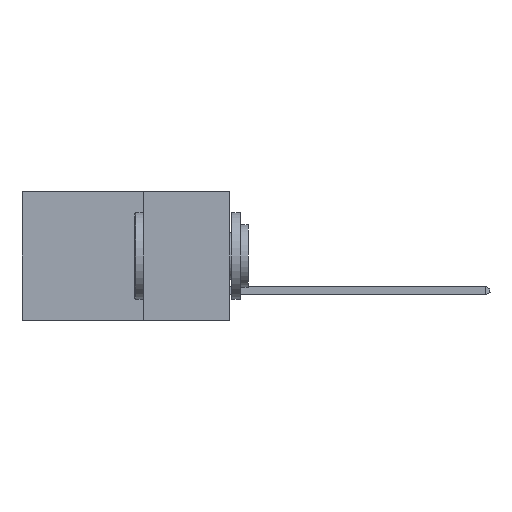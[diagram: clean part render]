
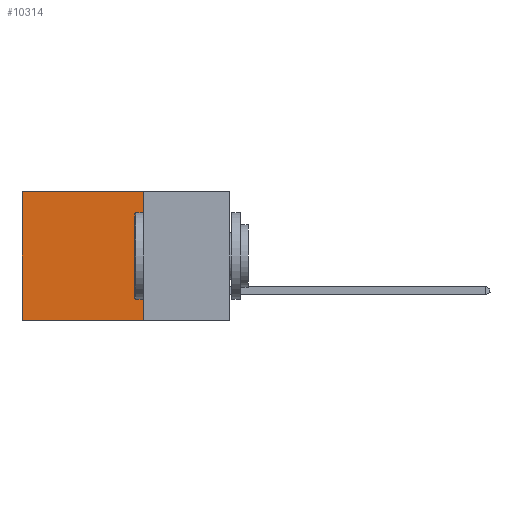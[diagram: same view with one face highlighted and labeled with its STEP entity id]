
A CAD part, left-side view. The second image highlights one B-rep face of the part: STEP entity #10314.
In plain terms, the highlighted planar face has unit normal (-1, 0, 0).
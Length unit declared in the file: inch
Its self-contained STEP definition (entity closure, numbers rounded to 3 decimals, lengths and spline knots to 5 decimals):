
#588 = VECTOR ( 'NONE', #27167, 39.37008 ) ;
#755 = ORIENTED_EDGE ( 'NONE', *, *, #18042, .F. ) ;
#1869 = CARTESIAN_POINT ( 'NONE',  ( 0.298, 0.25, 0. ) ) ;
#2701 = VECTOR ( 'NONE', #23231, 39.37008 ) ;
#3188 = VECTOR ( 'NONE', #9539, 39.37008 ) ;
#3940 = EDGE_LOOP ( 'NONE', ( #19233, #11216, #755, #17115 ) ) ;
#4338 = FACE_OUTER_BOUND ( 'NONE', #3940, .T. ) ;
#6070 = VERTEX_POINT ( 'NONE', #16393 ) ;
#6581 = CARTESIAN_POINT ( 'NONE',  ( 0.298, 0.6, 0. ) ) ;
#7579 = EDGE_CURVE ( 'NONE', #9698, #6070, #18651, .T. ) ;
#8254 = DIRECTION ( 'NONE',  ( 0., 1., 0. ) ) ;
#8403 = VERTEX_POINT ( 'NONE', #13054 ) ;
#9539 = DIRECTION ( 'NONE',  ( 0., 0., -1. ) ) ;
#9698 = VERTEX_POINT ( 'NONE', #6581 ) ;
#10314 = ADVANCED_FACE ( 'NONE', ( #4338 ), #25247, .F. ) ;
#10959 = LINE ( 'NONE', #22891, #3188 ) ;
#11216 = ORIENTED_EDGE ( 'NONE', *, *, #16402, .F. ) ;
#12782 = EDGE_CURVE ( 'NONE', #8403, #9698, #26139, .T. ) ;
#13054 = CARTESIAN_POINT ( 'NONE',  ( 0.298, 0.25, 0. ) ) ;
#13550 = CARTESIAN_POINT ( 'NONE',  ( 0.298, 0.25, 0. ) ) ;
#16119 = CARTESIAN_POINT ( 'NONE',  ( 0.298, 0.25, -0.37 ) ) ;
#16393 = CARTESIAN_POINT ( 'NONE',  ( 0.298, 0.6, -0.37 ) ) ;
#16402 = EDGE_CURVE ( 'NONE', #25079, #6070, #20658, .T. ) ;
#17115 = ORIENTED_EDGE ( 'NONE', *, *, #12782, .T. ) ;
#18042 = EDGE_CURVE ( 'NONE', #8403, #25079, #10959, .T. ) ;
#18209 = DIRECTION ( 'NONE',  ( 1., 0., 0. ) ) ;
#18651 = LINE ( 'NONE', #20940, #2701 ) ;
#19233 = ORIENTED_EDGE ( 'NONE', *, *, #7579, .T. ) ;
#20658 = LINE ( 'NONE', #21806, #23162 ) ;
#20940 = CARTESIAN_POINT ( 'NONE',  ( 0.298, 0.6, 0. ) ) ;
#21806 = CARTESIAN_POINT ( 'NONE',  ( 0.298, 0.25, -0.37 ) ) ;
#22891 = CARTESIAN_POINT ( 'NONE',  ( 0.298, 0.25, 0. ) ) ;
#23162 = VECTOR ( 'NONE', #8254, 39.37008 ) ;
#23231 = DIRECTION ( 'NONE',  ( 0., 0., -1. ) ) ;
#25079 = VERTEX_POINT ( 'NONE', #16119 ) ;
#25141 = DIRECTION ( 'NONE',  ( 0., 0., -1. ) ) ;
#25247 = PLANE ( 'NONE',  #26930 ) ;
#26139 = LINE ( 'NONE', #1869, #588 ) ;
#26930 = AXIS2_PLACEMENT_3D ( 'NONE', #13550, #18209, #25141 ) ;
#27167 = DIRECTION ( 'NONE',  ( 0., 1., 0. ) ) ;
